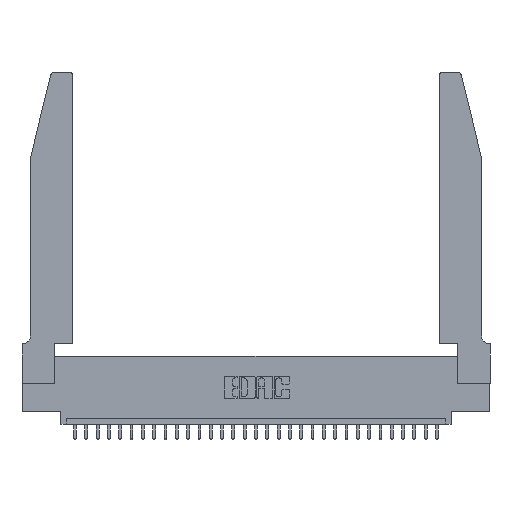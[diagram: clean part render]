
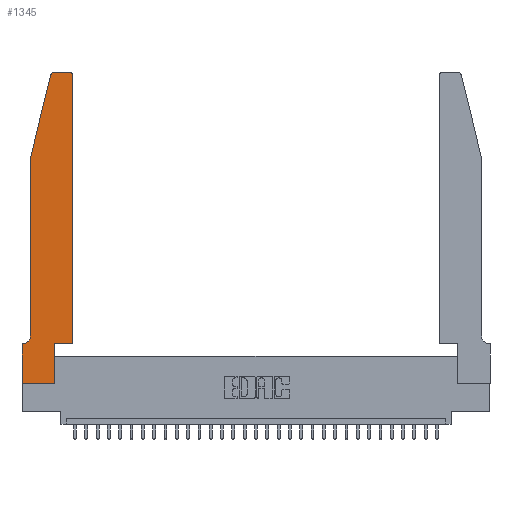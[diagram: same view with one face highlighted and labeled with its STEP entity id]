
A CAD part, top view. The second image highlights one B-rep face of the part: STEP entity #1345.
In plain terms, the highlighted planar face has unit normal (0, 0, 1).
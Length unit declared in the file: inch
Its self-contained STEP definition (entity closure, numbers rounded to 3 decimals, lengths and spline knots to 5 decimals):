
#173 = DIRECTION ( 'NONE',  ( 0., 0., 1. ) ) ;
#1345 = ADVANCED_FACE ( 'NONE', ( #15571 ), #21925, .T. ) ;
#1454 = ORIENTED_EDGE ( 'NONE', *, *, #18040, .T. ) ;
#1710 = VERTEX_POINT ( 'NONE', #14084 ) ;
#2296 = CARTESIAN_POINT ( 'NONE',  ( 0.0055, 0.42, 0.37 ) ) ;
#2297 = VECTOR ( 'NONE', #14877, 39.37008 ) ;
#2476 = EDGE_CURVE ( 'NONE', #20352, #23015, #28225, .T. ) ;
#3616 = LINE ( 'NONE', #14209, #28275 ) ;
#3633 = EDGE_CURVE ( 'NONE', #23015, #17237, #18594, .T. ) ;
#3904 = EDGE_CURVE ( 'NONE', #16590, #22161, #3616, .T. ) ;
#4114 = AXIS2_PLACEMENT_3D ( 'NONE', #7594, #173, #19651 ) ;
#4540 = LINE ( 'NONE', #29680, #2297 ) ;
#4599 = DIRECTION ( 'NONE',  ( 0., 0., -1. ) ) ;
#4818 = DIRECTION ( 'NONE',  ( 0., -1., 0. ) ) ;
#4925 = EDGE_CURVE ( 'NONE', #30657, #18997, #16318, .T. ) ;
#5324 = DIRECTION ( 'NONE',  ( 0., 0., 1. ) ) ;
#6283 = CARTESIAN_POINT ( 'NONE',  ( 0.0755, 0.35, 0.37 ) ) ;
#6378 = AXIS2_PLACEMENT_3D ( 'NONE', #2296, #4599, #14439 ) ;
#6944 = AXIS2_PLACEMENT_3D ( 'NONE', #29025, #5324, #7712 ) ;
#7209 = VERTEX_POINT ( 'NONE', #19788 ) ;
#7457 = EDGE_CURVE ( 'NONE', #18997, #1710, #4540, .T. ) ;
#7594 = CARTESIAN_POINT ( 'NONE',  ( 0., 0.35, 0.37 ) ) ;
#7669 = CARTESIAN_POINT ( 'NONE',  ( 0.4505, 0.35, 0.37 ) ) ;
#7712 = DIRECTION ( 'NONE',  ( 1., 0., 0. ) ) ;
#7856 = CARTESIAN_POINT ( 'NONE',  ( 0.284, 2.75, 0.37 ) ) ;
#10940 = ORIENTED_EDGE ( 'NONE', *, *, #30893, .T. ) ;
#11071 = CARTESIAN_POINT ( 'NONE',  ( 0.4505, 0.35, 0.37 ) ) ;
#11109 = VECTOR ( 'NONE', #27813, 39.37008 ) ;
#11189 = VERTEX_POINT ( 'NONE', #17096 ) ;
#11417 = CARTESIAN_POINT ( 'NONE',  ( 0.4205, 2.75, 0.37 ) ) ;
#11461 = ORIENTED_EDGE ( 'NONE', *, *, #25843, .T. ) ;
#11518 = LINE ( 'NONE', #6283, #17596 ) ;
#11573 = CIRCLE ( 'NONE', #18843, 0.03 ) ;
#11655 = LINE ( 'NONE', #28349, #23645 ) ;
#11885 = VECTOR ( 'NONE', #4818, 39.37008 ) ;
#12423 = ORIENTED_EDGE ( 'NONE', *, *, #4925, .T. ) ;
#12922 = ORIENTED_EDGE ( 'NONE', *, *, #27998, .T. ) ;
#14084 = CARTESIAN_POINT ( 'NONE',  ( 0.0755, 0.42, 0.37 ) ) ;
#14209 = CARTESIAN_POINT ( 'NONE',  ( 0.2605, 2.75, 0.37 ) ) ;
#14335 = CARTESIAN_POINT ( 'NONE',  ( 0., 0., 0.37 ) ) ;
#14439 = DIRECTION ( 'NONE',  ( -1., 0., 0. ) ) ;
#14790 = EDGE_LOOP ( 'NONE', ( #19893, #15218, #12423, #22197, #12922, #11461, #26213, #10940, #27247, #22609, #22726, #1454 ) ) ;
#14877 = DIRECTION ( 'NONE',  ( 0., -1., 0. ) ) ;
#15218 = ORIENTED_EDGE ( 'NONE', *, *, #20123, .T. ) ;
#15571 = FACE_OUTER_BOUND ( 'NONE', #14790, .T. ) ;
#15881 = CARTESIAN_POINT ( 'NONE',  ( 0.284, 2.72, 0.37 ) ) ;
#16318 = LINE ( 'NONE', #25097, #24895 ) ;
#16590 = VERTEX_POINT ( 'NONE', #11417 ) ;
#17096 = CARTESIAN_POINT ( 'NONE',  ( 0.0055, 0.35, 0.37 ) ) ;
#17237 = VERTEX_POINT ( 'NONE', #20767 ) ;
#17596 = VECTOR ( 'NONE', #20325, 39.37008 ) ;
#17756 = CIRCLE ( 'NONE', #6944, 0.03 ) ;
#18040 = EDGE_CURVE ( 'NONE', #17237, #16590, #17756, .T. ) ;
#18594 = LINE ( 'NONE', #11071, #11109 ) ;
#18843 = AXIS2_PLACEMENT_3D ( 'NONE', #15881, #22759, #27587 ) ;
#18997 = VERTEX_POINT ( 'NONE', #19762 ) ;
#19197 = DIRECTION ( 'NONE',  ( 1., 0., 0. ) ) ;
#19220 = VERTEX_POINT ( 'NONE', #25663 ) ;
#19651 = DIRECTION ( 'NONE',  ( 1., 0., 0. ) ) ;
#19762 = CARTESIAN_POINT ( 'NONE',  ( 0.0755, 2., 0.37 ) ) ;
#19788 = CARTESIAN_POINT ( 'NONE',  ( 0., 0.35, 0.37 ) ) ;
#19893 = ORIENTED_EDGE ( 'NONE', *, *, #3904, .T. ) ;
#20123 = EDGE_CURVE ( 'NONE', #22161, #30657, #11573, .T. ) ;
#20325 = DIRECTION ( 'NONE',  ( -1., 0., 0. ) ) ;
#20352 = VERTEX_POINT ( 'NONE', #26301 ) ;
#20465 = VERTEX_POINT ( 'NONE', #28856 ) ;
#20671 = CARTESIAN_POINT ( 'NONE',  ( 0.25487, 2.72718, 0.37 ) ) ;
#20767 = CARTESIAN_POINT ( 'NONE',  ( 0.4505, 2.72, 0.37 ) ) ;
#21617 = LINE ( 'NONE', #14335, #11885 ) ;
#21912 = DIRECTION ( 'NONE',  ( -1., 0., 0. ) ) ;
#21925 = PLANE ( 'NONE',  #4114 ) ;
#22161 = VERTEX_POINT ( 'NONE', #7856 ) ;
#22197 = ORIENTED_EDGE ( 'NONE', *, *, #7457, .T. ) ;
#22609 = ORIENTED_EDGE ( 'NONE', *, *, #2476, .T. ) ;
#22726 = ORIENTED_EDGE ( 'NONE', *, *, #3633, .T. ) ;
#22759 = DIRECTION ( 'NONE',  ( 0., 0., 1. ) ) ;
#23015 = VERTEX_POINT ( 'NONE', #24787 ) ;
#23645 = VECTOR ( 'NONE', #19197, 39.37008 ) ;
#23964 = CARTESIAN_POINT ( 'NONE',  ( 0.2865, 0.35, 0.37 ) ) ;
#24110 = VECTOR ( 'NONE', #25411, 39.37008 ) ;
#24787 = CARTESIAN_POINT ( 'NONE',  ( 0.4505, 0.35, 0.37 ) ) ;
#24895 = VECTOR ( 'NONE', #27294, 39.37008 ) ;
#25097 = CARTESIAN_POINT ( 'NONE',  ( 0.0755, 2., 0.37 ) ) ;
#25411 = DIRECTION ( 'NONE',  ( 1., 0., 0. ) ) ;
#25663 = CARTESIAN_POINT ( 'NONE',  ( 0.2865, 0., 0.37 ) ) ;
#25843 = EDGE_CURVE ( 'NONE', #11189, #7209, #11518, .T. ) ;
#26040 = DIRECTION ( 'NONE',  ( 0., 1., 0. ) ) ;
#26087 = EDGE_CURVE ( 'NONE', #7209, #20465, #21617, .T. ) ;
#26213 = ORIENTED_EDGE ( 'NONE', *, *, #26087, .T. ) ;
#26301 = CARTESIAN_POINT ( 'NONE',  ( 0.2865, 0.35, 0.37 ) ) ;
#26346 = EDGE_CURVE ( 'NONE', #19220, #20352, #28672, .T. ) ;
#27247 = ORIENTED_EDGE ( 'NONE', *, *, #26346, .T. ) ;
#27294 = DIRECTION ( 'NONE',  ( -0.239, -0.971, 0. ) ) ;
#27587 = DIRECTION ( 'NONE',  ( 1., 0., 0. ) ) ;
#27813 = DIRECTION ( 'NONE',  ( 0., 1., 0. ) ) ;
#27998 = EDGE_CURVE ( 'NONE', #1710, #11189, #28953, .T. ) ;
#28225 = LINE ( 'NONE', #7669, #24110 ) ;
#28275 = VECTOR ( 'NONE', #21912, 39.37008 ) ;
#28317 = VECTOR ( 'NONE', #26040, 39.37008 ) ;
#28349 = CARTESIAN_POINT ( 'NONE',  ( 0., 0., 0.37 ) ) ;
#28672 = LINE ( 'NONE', #23964, #28317 ) ;
#28856 = CARTESIAN_POINT ( 'NONE',  ( 0., 0., 0.37 ) ) ;
#28953 = CIRCLE ( 'NONE', #6378, 0.07 ) ;
#29025 = CARTESIAN_POINT ( 'NONE',  ( 0.4205, 2.72, 0.37 ) ) ;
#29680 = CARTESIAN_POINT ( 'NONE',  ( 0.0755, 2., 0.37 ) ) ;
#30657 = VERTEX_POINT ( 'NONE', #20671 ) ;
#30893 = EDGE_CURVE ( 'NONE', #20465, #19220, #11655, .T. ) ;
